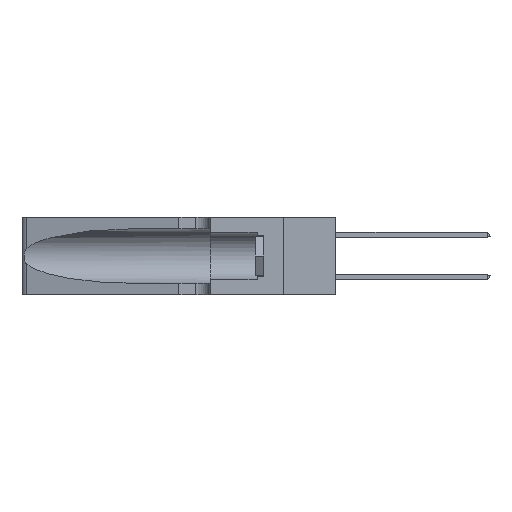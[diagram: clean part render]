
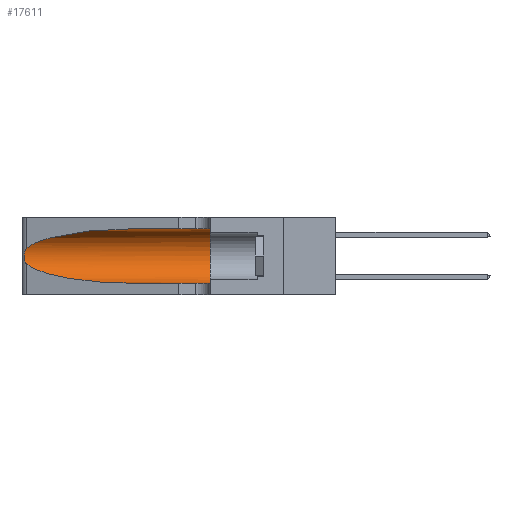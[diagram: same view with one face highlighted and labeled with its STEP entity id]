
A CAD part, left-side view. The second image highlights one B-rep face of the part: STEP entity #17611.
In plain terms, the highlighted cylindrical face has radius 3.308 mm (diameter 6.617 mm), a partial arc.
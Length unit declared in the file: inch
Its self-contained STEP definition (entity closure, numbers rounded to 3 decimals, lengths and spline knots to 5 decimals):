
#81 = CARTESIAN_POINT ( 'NONE',  ( 0.25555, 1.22994, 0.2215 ) ) ;
#188 = CARTESIAN_POINT ( 'NONE',  ( 0.25639, 1.23186, 0.15144 ) ) ;
#337 = CARTESIAN_POINT ( 'NONE',  ( 0.1305, 1.61858, 0.185 ) ) ;
#808 = AXIS2_PLACEMENT_3D ( 'NONE', #337, #27827, #11853 ) ;
#2417 = CARTESIAN_POINT ( 'NONE',  ( 0.1305, 0.72297, 0.05475 ) ) ;
#2527 = CARTESIAN_POINT ( 'NONE',  ( 0.25487, 1.22718, 0.14631 ) ) ;
#2546 = EDGE_CURVE ( 'NONE', #22297, #11237, #24336, .T. ) ;
#2604 = EDGE_CURVE ( 'NONE', #24489, #22297, #28974, .T. ) ;
#3216 = CARTESIAN_POINT ( 'NONE',  ( 0.1305, 0.35, 0.05475 ) ) ;
#4800 = CARTESIAN_POINT ( 'NONE',  ( 0.25487, 1.22718, 0.22369 ) ) ;
#5426 = CARTESIAN_POINT ( 'NONE',  ( 0.25487, 1.22718, 0.22369 ) ) ;
#5497 = FACE_OUTER_BOUND ( 'NONE', #20060, .T. ) ;
#5831 = CARTESIAN_POINT ( 'NONE',  ( 0.18966, 0.96281, 0.05475 ) ) ;
#6336 = EDGE_CURVE ( 'NONE', #7866, #20099, #17373, .T. ) ;
#6384 = DIRECTION ( 'NONE',  ( 0., -1., 0. ) ) ;
#6484 = DIRECTION ( 'NONE',  ( 0., -1., 0. ) ) ;
#7125 = CARTESIAN_POINT ( 'NONE',  ( 0.25854, 1.2359, 0.20912 ) ) ;
#7622 = CARTESIAN_POINT ( 'NONE',  ( 0.18966, 0.96281, 0.31525 ) ) ;
#7813 = CARTESIAN_POINT ( 'NONE',  ( 0.1305, 0.35, 0.31525 ) ) ;
#7866 = VERTEX_POINT ( 'NONE', #19129 ) ;
#9401 = CARTESIAN_POINT ( 'NONE',  ( 0.26075, 1.23896, 0.19203 ) ) ;
#9408 = CYLINDRICAL_SURFACE ( 'NONE', #808, 0.13025 ) ;
#10520 = EDGE_CURVE ( 'NONE', #24489, #7866, #26512, .T. ) ;
#11237 = VERTEX_POINT ( 'NONE', #3216 ) ;
#11706 = CARTESIAN_POINT ( 'NONE',  ( 0.26017, 1.23833, 0.17102 ) ) ;
#11853 = DIRECTION ( 'NONE',  ( 0., 0., -1. ) ) ;
#12263 = LINE ( 'NONE', #22363, #14668 ) ;
#13182 = CARTESIAN_POINT ( 'NONE',  ( 0.1305, 0.35, 0.185 ) ) ;
#14023 = CARTESIAN_POINT ( 'NONE',  ( 0.25789, 1.23486, 0.15765 ) ) ;
#14668 = VECTOR ( 'NONE', #6384, 39.37008 ) ;
#14690 = ORIENTED_EDGE ( 'NONE', *, *, #6336, .T. ) ;
#15485 = DIRECTION ( 'NONE',  ( 0., 0., 1. ) ) ;
#16330 = CARTESIAN_POINT ( 'NONE',  ( 0.25555, 1.22993, 0.14849 ) ) ;
#16498 = EDGE_CURVE ( 'NONE', #20099, #24236, #24664, .T. ) ;
#16843 = ORIENTED_EDGE ( 'NONE', *, *, #2546, .F. ) ;
#16848 = VECTOR ( 'NONE', #6484, 39.37008 ) ;
#17222 = CARTESIAN_POINT ( 'NONE',  ( 0.25487, 1.22718, 0.14631 ) ) ;
#17373 = B_SPLINE_CURVE_WITH_KNOTS ( 'NONE', 3,
 ( #4800, #81, #27586, #20793, #7125, #23098, #9401, #25386, #11706, #27680, #14023, #188, #16330, #2527 ),
 .UNSPECIFIED., .F., .F.,
 ( 4, 2, 2, 2, 2, 2, 4 ),
 ( 0., 0.00027, 0.00053, 0.00107, 0.0016, 0.00187, 0.00214 ),
 .UNSPECIFIED. ) ;
#17611 = ADVANCED_FACE ( 'NONE', ( #5497 ), #9408, .F. ) ;
#17881 = CARTESIAN_POINT ( 'NONE',  ( 0.1305, 1.61858, 0.31525 ) ) ;
#19119 = CARTESIAN_POINT ( 'NONE',  ( 0.2373, 1.15595, 0.28018 ) ) ;
#19129 = CARTESIAN_POINT ( 'NONE',  ( 0.25487, 1.22718, 0.22369 ) ) ;
#19318 = ORIENTED_EDGE ( 'NONE', *, *, #10520, .T. ) ;
#19511 = CARTESIAN_POINT ( 'NONE',  ( 0.2373, 1.15595, 0.08982 ) ) ;
#20060 = EDGE_LOOP ( 'NONE', ( #19318, #14690, #26822, #28257, #16843, #22891 ) ) ;
#20099 = VERTEX_POINT ( 'NONE', #22517 ) ;
#20793 = CARTESIAN_POINT ( 'NONE',  ( 0.25787, 1.23484, 0.2124 ) ) ;
#21481 = CARTESIAN_POINT ( 'NONE',  ( 0.1305, 0.72297, 0.31525 ) ) ;
#21806 = CARTESIAN_POINT ( 'NONE',  ( 0.1305, 0.72297, 0.05475 ) ) ;
#22297 = VERTEX_POINT ( 'NONE', #7813 ) ;
#22363 = CARTESIAN_POINT ( 'NONE',  ( 0.1305, 1.61858, 0.05475 ) ) ;
#22517 = CARTESIAN_POINT ( 'NONE',  ( 0.25487, 1.22718, 0.14631 ) ) ;
#22891 = ORIENTED_EDGE ( 'NONE', *, *, #2604, .F. ) ;
#23098 = CARTESIAN_POINT ( 'NONE',  ( 0.26018, 1.23835, 0.19895 ) ) ;
#23173 = EDGE_CURVE ( 'NONE', #24236, #11237, #12263, .T. ) ;
#23614 = CARTESIAN_POINT ( 'NONE',  ( 0.1305, 0.72297, 0.31525 ) ) ;
#23841 = AXIS2_PLACEMENT_3D ( 'NONE', #13182, #29152, #15485 ) ;
#24236 = VERTEX_POINT ( 'NONE', #2417 ) ;
#24336 = CIRCLE ( 'NONE', #23841, 0.13025 ) ;
#24489 = VERTEX_POINT ( 'NONE', #21481 ) ;
#24664 =( BOUNDED_CURVE ( )  B_SPLINE_CURVE ( 3, ( #17222, #19511, #5831, #21806 ),
 .UNSPECIFIED., .F., .T. ) 
 B_SPLINE_CURVE_WITH_KNOTS ( ( 4, 4 ),
 ( 3.44316, 4.71239 ),
 .UNSPECIFIED. ) 
 CURVE ( )  GEOMETRIC_REPRESENTATION_ITEM ( )  RATIONAL_B_SPLINE_CURVE ( ( 1., 0.87, 0.87, 1. ) ) 
 REPRESENTATION_ITEM ( '' )  );
#25386 = CARTESIAN_POINT ( 'NONE',  ( 0.26075, 1.23896, 0.178 ) ) ;
#26512 =( BOUNDED_CURVE ( )  B_SPLINE_CURVE ( 3, ( #23614, #7622, #19119, #5426 ),
 .UNSPECIFIED., .F., .F. ) 
 B_SPLINE_CURVE_WITH_KNOTS ( ( 4, 4 ),
 ( 1.5708, 2.84003 ),
 .UNSPECIFIED. ) 
 CURVE ( )  GEOMETRIC_REPRESENTATION_ITEM ( )  RATIONAL_B_SPLINE_CURVE ( ( 1., 0.87, 0.87, 1. ) ) 
 REPRESENTATION_ITEM ( '' )  );
#26822 = ORIENTED_EDGE ( 'NONE', *, *, #16498, .T. ) ;
#27586 = CARTESIAN_POINT ( 'NONE',  ( 0.25639, 1.23184, 0.21858 ) ) ;
#27680 = CARTESIAN_POINT ( 'NONE',  ( 0.25856, 1.23593, 0.16098 ) ) ;
#27827 = DIRECTION ( 'NONE',  ( 0., -1., 0. ) ) ;
#28257 = ORIENTED_EDGE ( 'NONE', *, *, #23173, .T. ) ;
#28974 = LINE ( 'NONE', #17881, #16848 ) ;
#29152 = DIRECTION ( 'NONE',  ( 0., 1., 0. ) ) ;
